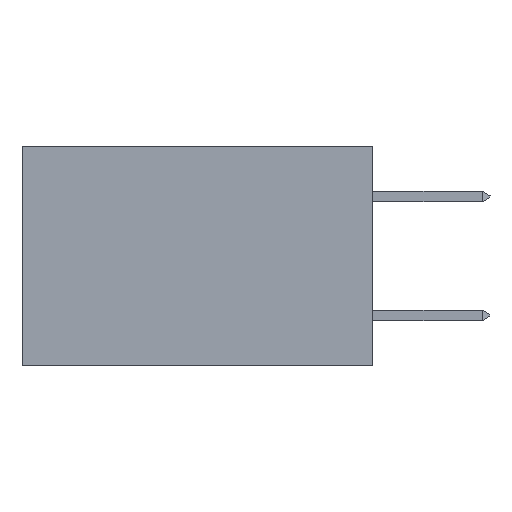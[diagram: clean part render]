
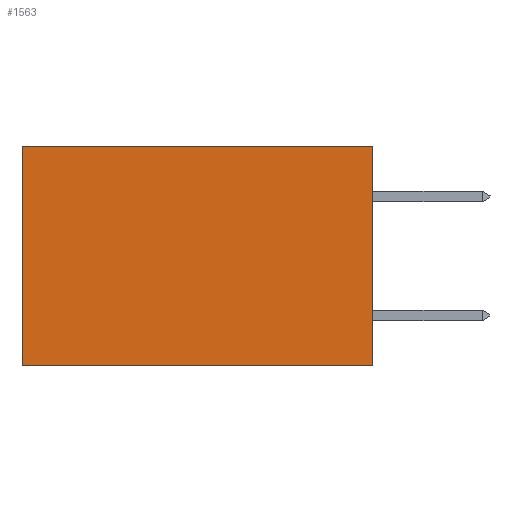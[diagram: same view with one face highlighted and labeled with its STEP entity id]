
A CAD part, left-side view. The second image highlights one B-rep face of the part: STEP entity #1563.
In plain terms, the highlighted planar face has unit normal (-1, 0, 0).
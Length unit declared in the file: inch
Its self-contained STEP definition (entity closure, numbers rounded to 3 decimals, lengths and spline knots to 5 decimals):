
#94 = LINE ( 'NONE', #10204, #14348 ) ;
#913 = CARTESIAN_POINT ( 'NONE',  ( 0.277, 0., -0.37 ) ) ;
#988 = DIRECTION ( 'NONE',  ( 0., 0., -1. ) ) ;
#1096 = LINE ( 'NONE', #11525, #12648 ) ;
#1116 = DIRECTION ( 'NONE',  ( 0., 0., -1. ) ) ;
#1144 = VERTEX_POINT ( 'NONE', #913 ) ;
#1563 = ADVANCED_FACE ( 'NONE', ( #8396 ), #7318, .F. ) ;
#1888 = VECTOR ( 'NONE', #1116, 39.37008 ) ;
#1949 = ORIENTED_EDGE ( 'NONE', *, *, #7828, .T. ) ;
#2301 = CARTESIAN_POINT ( 'NONE',  ( 0.277, 0., -0.37 ) ) ;
#2388 = LINE ( 'NONE', #11616, #9271 ) ;
#2421 = CARTESIAN_POINT ( 'NONE',  ( 0.277, 0.59, -0.37 ) ) ;
#3146 = EDGE_CURVE ( 'NONE', #1144, #6044, #94, .T. ) ;
#5135 = AXIS2_PLACEMENT_3D ( 'NONE', #13626, #13685, #988 ) ;
#5883 = DIRECTION ( 'NONE',  ( 0., 0., -1. ) ) ;
#6044 = VERTEX_POINT ( 'NONE', #2421 ) ;
#7255 = EDGE_CURVE ( 'NONE', #12234, #6044, #2388, .T. ) ;
#7311 = VERTEX_POINT ( 'NONE', #12789 ) ;
#7318 = PLANE ( 'NONE',  #5135 ) ;
#7790 = ORIENTED_EDGE ( 'NONE', *, *, #14912, .F. ) ;
#7828 = EDGE_CURVE ( 'NONE', #7311, #12234, #1096, .T. ) ;
#8074 = LINE ( 'NONE', #2301, #1888 ) ;
#8396 = FACE_OUTER_BOUND ( 'NONE', #12690, .T. ) ;
#9271 = VECTOR ( 'NONE', #5883, 39.37008 ) ;
#9324 = DIRECTION ( 'NONE',  ( 0., 1., 0. ) ) ;
#10204 = CARTESIAN_POINT ( 'NONE',  ( 0.277, 0., -0.37 ) ) ;
#10301 = DIRECTION ( 'NONE',  ( 0., 1., 0. ) ) ;
#10450 = CARTESIAN_POINT ( 'NONE',  ( 0.277, 0.59, 0. ) ) ;
#11525 = CARTESIAN_POINT ( 'NONE',  ( 0.277, 0., 0. ) ) ;
#11616 = CARTESIAN_POINT ( 'NONE',  ( 0.277, 0.59, -0.37 ) ) ;
#12234 = VERTEX_POINT ( 'NONE', #10450 ) ;
#12648 = VECTOR ( 'NONE', #9324, 39.37008 ) ;
#12690 = EDGE_LOOP ( 'NONE', ( #12724, #13078, #7790, #1949 ) ) ;
#12724 = ORIENTED_EDGE ( 'NONE', *, *, #7255, .T. ) ;
#12789 = CARTESIAN_POINT ( 'NONE',  ( 0.277, 0., 0. ) ) ;
#13078 = ORIENTED_EDGE ( 'NONE', *, *, #3146, .F. ) ;
#13626 = CARTESIAN_POINT ( 'NONE',  ( 0.277, 0., -0.37 ) ) ;
#13685 = DIRECTION ( 'NONE',  ( 1., 0., 0. ) ) ;
#14348 = VECTOR ( 'NONE', #10301, 39.37008 ) ;
#14912 = EDGE_CURVE ( 'NONE', #7311, #1144, #8074, .T. ) ;
